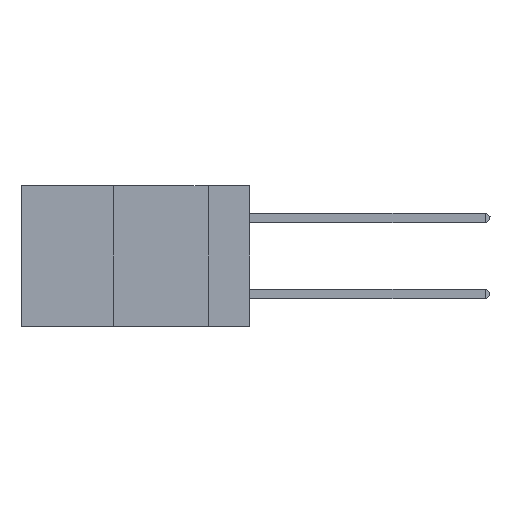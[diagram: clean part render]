
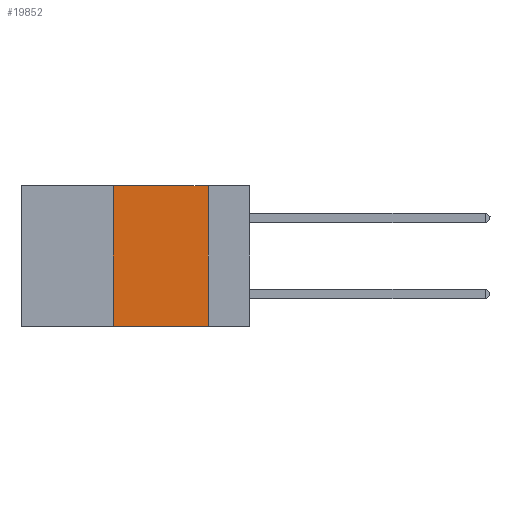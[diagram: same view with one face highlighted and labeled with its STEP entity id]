
A CAD part, left-side view. The second image highlights one B-rep face of the part: STEP entity #19852.
In plain terms, the highlighted planar face has unit normal (-1, 0, 0).
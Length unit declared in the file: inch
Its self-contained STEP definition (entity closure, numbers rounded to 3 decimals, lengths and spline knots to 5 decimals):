
#139 = VERTEX_POINT ( 'NONE', #8989 ) ;
#916 = AXIS2_PLACEMENT_3D ( 'NONE', #13154, #23541, #11086 ) ;
#3159 = EDGE_LOOP ( 'NONE', ( #6360, #7082, #18246, #11959 ) ) ;
#5185 = PLANE ( 'NONE',  #916 ) ;
#5318 = CARTESIAN_POINT ( 'NONE',  ( 0., 0.11, -0.37 ) ) ;
#6360 = ORIENTED_EDGE ( 'NONE', *, *, #26888, .F. ) ;
#7082 = ORIENTED_EDGE ( 'NONE', *, *, #22764, .F. ) ;
#8059 = LINE ( 'NONE', #16535, #22354 ) ;
#8989 = CARTESIAN_POINT ( 'NONE',  ( 0., 0.11, 0. ) ) ;
#9034 = VECTOR ( 'NONE', #22545, 39.37008 ) ;
#10268 = CARTESIAN_POINT ( 'NONE',  ( 0., 0.36, 0. ) ) ;
#11086 = DIRECTION ( 'NONE',  ( 0., 0., -1. ) ) ;
#11931 = DIRECTION ( 'NONE',  ( 0., -1., 0. ) ) ;
#11959 = ORIENTED_EDGE ( 'NONE', *, *, #18223, .T. ) ;
#13154 = CARTESIAN_POINT ( 'NONE',  ( 0., 0.6, 0. ) ) ;
#14218 = CARTESIAN_POINT ( 'NONE',  ( 0., 0.11, 0. ) ) ;
#14399 = LINE ( 'NONE', #10268, #17105 ) ;
#16535 = CARTESIAN_POINT ( 'NONE',  ( 0., 0.6, 0. ) ) ;
#17105 = VECTOR ( 'NONE', #18737, 39.37008 ) ;
#18223 = EDGE_CURVE ( 'NONE', #25940, #18726, #19983, .T. ) ;
#18246 = ORIENTED_EDGE ( 'NONE', *, *, #22368, .F. ) ;
#18726 = VERTEX_POINT ( 'NONE', #5318 ) ;
#18737 = DIRECTION ( 'NONE',  ( 0., 0., 1. ) ) ;
#19832 = FACE_OUTER_BOUND ( 'NONE', #3159, .T. ) ;
#19852 = ADVANCED_FACE ( 'NONE', ( #19832 ), #5185, .F. ) ;
#19983 = LINE ( 'NONE', #20525, #26654 ) ;
#20525 = CARTESIAN_POINT ( 'NONE',  ( 0., 0.6, -0.37 ) ) ;
#21100 = CARTESIAN_POINT ( 'NONE',  ( 0., 0.36, -0.37 ) ) ;
#22354 = VECTOR ( 'NONE', #26953, 39.37008 ) ;
#22368 = EDGE_CURVE ( 'NONE', #25940, #25109, #14399, .T. ) ;
#22545 = DIRECTION ( 'NONE',  ( 0., 0., -1. ) ) ;
#22764 = EDGE_CURVE ( 'NONE', #25109, #139, #8059, .T. ) ;
#23541 = DIRECTION ( 'NONE',  ( 1., 0., 0. ) ) ;
#25109 = VERTEX_POINT ( 'NONE', #26705 ) ;
#25940 = VERTEX_POINT ( 'NONE', #21100 ) ;
#26654 = VECTOR ( 'NONE', #11931, 39.37008 ) ;
#26705 = CARTESIAN_POINT ( 'NONE',  ( 0., 0.36, 0. ) ) ;
#26807 = LINE ( 'NONE', #14218, #9034 ) ;
#26888 = EDGE_CURVE ( 'NONE', #139, #18726, #26807, .T. ) ;
#26953 = DIRECTION ( 'NONE',  ( 0., -1., 0. ) ) ;
